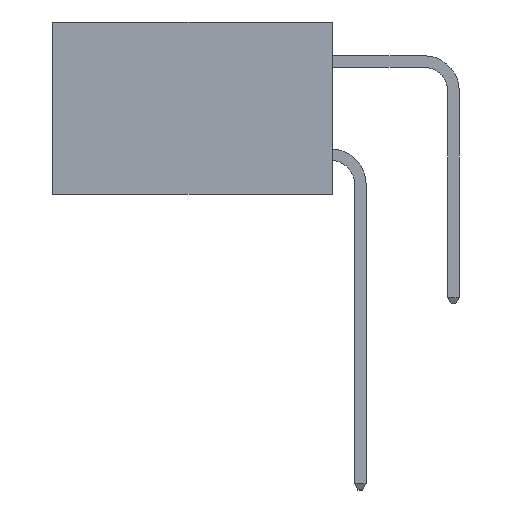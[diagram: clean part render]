
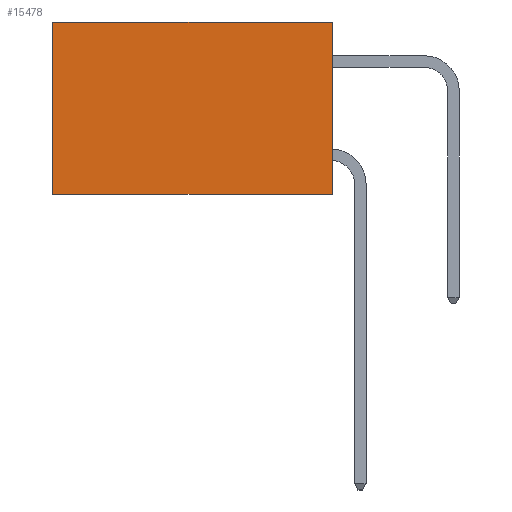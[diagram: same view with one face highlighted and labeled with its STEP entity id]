
A CAD part, left-side view. The second image highlights one B-rep face of the part: STEP entity #15478.
In plain terms, the highlighted planar face has unit normal (-1, 0, 0).
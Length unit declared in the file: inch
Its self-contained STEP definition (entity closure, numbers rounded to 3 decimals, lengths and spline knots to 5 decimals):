
#1070 = ORIENTED_EDGE ( 'NONE', *, *, #9080, .T. ) ;
#1924 = VECTOR ( 'NONE', #15251, 39.37008 ) ;
#2019 = CARTESIAN_POINT ( 'NONE',  ( 0.2615, 0., -0.37 ) ) ;
#2292 = CARTESIAN_POINT ( 'NONE',  ( 0.2615, 0.6, -0.37 ) ) ;
#2320 = EDGE_LOOP ( 'NONE', ( #6240, #16906, #5377, #1070 ) ) ;
#2823 = LINE ( 'NONE', #16138, #6966 ) ;
#2948 = CARTESIAN_POINT ( 'NONE',  ( 0.2615, 0.6, 0. ) ) ;
#4251 = VERTEX_POINT ( 'NONE', #2292 ) ;
#4643 = EDGE_CURVE ( 'NONE', #7266, #4251, #2823, .T. ) ;
#5377 = ORIENTED_EDGE ( 'NONE', *, *, #12392, .F. ) ;
#5927 = LINE ( 'NONE', #9037, #15702 ) ;
#6135 = VERTEX_POINT ( 'NONE', #8830 ) ;
#6240 = ORIENTED_EDGE ( 'NONE', *, *, #15454, .T. ) ;
#6509 = LINE ( 'NONE', #13842, #1924 ) ;
#6966 = VECTOR ( 'NONE', #16011, 39.37008 ) ;
#7266 = VERTEX_POINT ( 'NONE', #2019 ) ;
#8830 = CARTESIAN_POINT ( 'NONE',  ( 0.2615, 0., 0. ) ) ;
#9033 = DIRECTION ( 'NONE',  ( 0., 1., 0. ) ) ;
#9037 = CARTESIAN_POINT ( 'NONE',  ( 0.2615, 0., 0. ) ) ;
#9079 = VECTOR ( 'NONE', #11474, 39.37008 ) ;
#9080 = EDGE_CURVE ( 'NONE', #6135, #9376, #5927, .T. ) ;
#9376 = VERTEX_POINT ( 'NONE', #2948 ) ;
#10020 = DIRECTION ( 'NONE',  ( 0., 0., -1. ) ) ;
#10051 = DIRECTION ( 'NONE',  ( 1., 0., 0. ) ) ;
#10111 = CARTESIAN_POINT ( 'NONE',  ( 0.2615, 0., -0.37 ) ) ;
#11098 = PLANE ( 'NONE',  #12661 ) ;
#11359 = FACE_OUTER_BOUND ( 'NONE', #2320, .T. ) ;
#11474 = DIRECTION ( 'NONE',  ( 0., 0., -1. ) ) ;
#11562 = CARTESIAN_POINT ( 'NONE',  ( 0.2615, 0.6, -0.37 ) ) ;
#12392 = EDGE_CURVE ( 'NONE', #6135, #7266, #6509, .T. ) ;
#12661 = AXIS2_PLACEMENT_3D ( 'NONE', #10111, #10051, #10020 ) ;
#13842 = CARTESIAN_POINT ( 'NONE',  ( 0.2615, 0., -0.37 ) ) ;
#15251 = DIRECTION ( 'NONE',  ( 0., 0., -1. ) ) ;
#15454 = EDGE_CURVE ( 'NONE', #9376, #4251, #15559, .T. ) ;
#15478 = ADVANCED_FACE ( 'NONE', ( #11359 ), #11098, .F. ) ;
#15559 = LINE ( 'NONE', #11562, #9079 ) ;
#15702 = VECTOR ( 'NONE', #9033, 39.37008 ) ;
#16011 = DIRECTION ( 'NONE',  ( 0., 1., 0. ) ) ;
#16138 = CARTESIAN_POINT ( 'NONE',  ( 0.2615, 0., -0.37 ) ) ;
#16906 = ORIENTED_EDGE ( 'NONE', *, *, #4643, .F. ) ;
